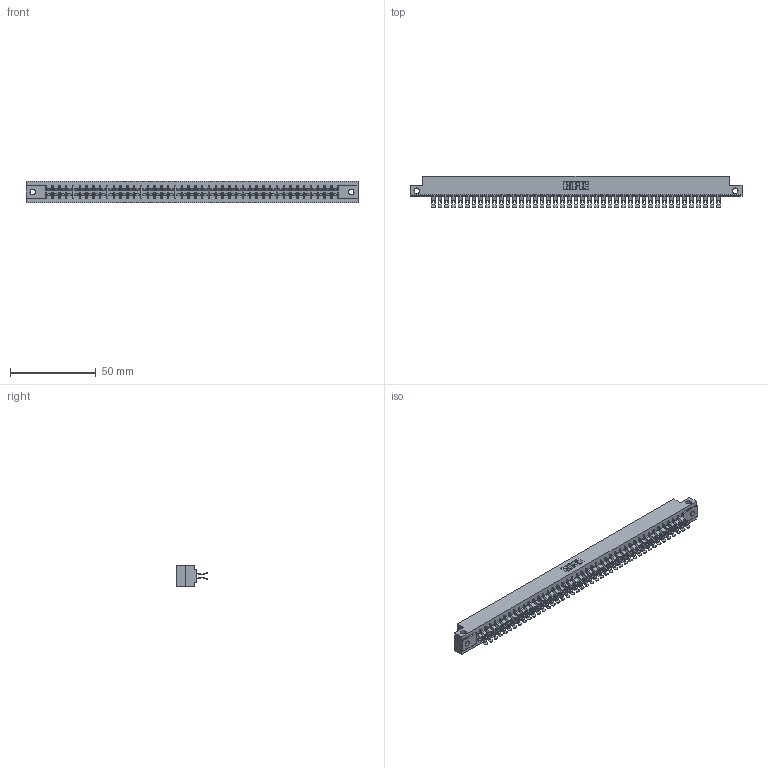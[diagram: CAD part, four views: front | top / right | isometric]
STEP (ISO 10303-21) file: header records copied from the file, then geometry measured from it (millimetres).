
FILE_DESCRIPTION (( 'STEP AP203' ), '1' );
FILE_NAME ('355-086-555-212.STEP', '2020-09-20T11:11:54', ( '' ), ( '' ), 'SwSTEP 2.0', 'SolidWorks 2020', '' );
FILE_SCHEMA (( 'CONFIG_CONTROL_DESIGN' ));
Length unit declared in the file: inch
Products named in the file (3): 355-086-555-212; 305 Part_.128 Dia; 305-290-001_555
Assembly tree (87 placements, depth 2):
  355-086-555-212
    305 Part_.128 Dia
    305-290-001_555  x86
Bounding box: 193.4 x 18.41 x 12.7 mm (x, y, z)
Volume: 20227.1 mm3; surface area: 27470.4 mm2
Topology: 87 solids, 87 shells, 5804 faces, 17337 edges, 11322 vertices
Faces by surface type: plane 2820, cylinder 2812, sphere 172
Entity records: 47466 total; most frequent: CARTESIAN_POINT 7921, ORIENTED_EDGE 7810, DIRECTION 7595, EDGE_CURVE 3905, LINE 3123, VECTOR 3123, VERTEX_POINT 2482, AXIS2_PLACEMENT_3D 2236
